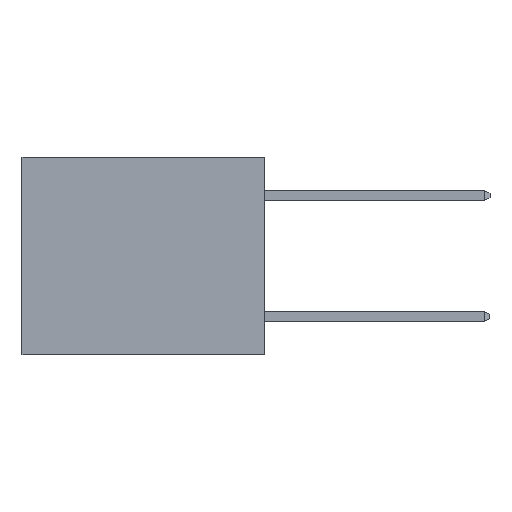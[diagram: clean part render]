
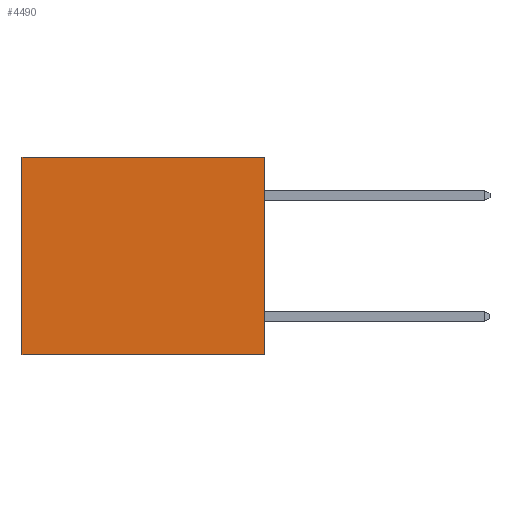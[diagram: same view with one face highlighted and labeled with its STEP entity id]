
A CAD part, left-side view. The second image highlights one B-rep face of the part: STEP entity #4490.
In plain terms, the highlighted planar face has unit normal (-1, 0, 0).
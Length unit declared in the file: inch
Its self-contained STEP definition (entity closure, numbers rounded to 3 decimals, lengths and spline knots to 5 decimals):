
#353 = CARTESIAN_POINT ( 'NONE',  ( 0.3165, 0., -0.49 ) ) ;
#411 = FACE_OUTER_BOUND ( 'NONE', #10438, .T. ) ;
#533 = EDGE_CURVE ( 'NONE', #697, #10059, #6266, .T. ) ;
#611 = AXIS2_PLACEMENT_3D ( 'NONE', #3777, #4558, #1979 ) ;
#697 = VERTEX_POINT ( 'NONE', #9895 ) ;
#712 = DIRECTION ( 'NONE',  ( 0., 1., 0. ) ) ;
#1979 = DIRECTION ( 'NONE',  ( 0., 0., -1. ) ) ;
#2061 = DIRECTION ( 'NONE',  ( 0., 0., -1. ) ) ;
#2136 = VECTOR ( 'NONE', #2906, 39.37008 ) ;
#2797 = CARTESIAN_POINT ( 'NONE',  ( 0.3165, 0.6, 0. ) ) ;
#2906 = DIRECTION ( 'NONE',  ( 0., 1., 0. ) ) ;
#2967 = PLANE ( 'NONE',  #611 ) ;
#3192 = LINE ( 'NONE', #7329, #3478 ) ;
#3478 = VECTOR ( 'NONE', #2061, 39.37008 ) ;
#3777 = CARTESIAN_POINT ( 'NONE',  ( 0.3165, 0., -0.49 ) ) ;
#3901 = VECTOR ( 'NONE', #712, 39.37008 ) ;
#4215 = ORIENTED_EDGE ( 'NONE', *, *, #11050, .T. ) ;
#4490 = ADVANCED_FACE ( 'NONE', ( #411 ), #2967, .F. ) ;
#4558 = DIRECTION ( 'NONE',  ( 1., 0., 0. ) ) ;
#4813 = VERTEX_POINT ( 'NONE', #8551 ) ;
#5181 = LINE ( 'NONE', #7562, #5321 ) ;
#5243 = ORIENTED_EDGE ( 'NONE', *, *, #533, .T. ) ;
#5321 = VECTOR ( 'NONE', #7449, 39.37008 ) ;
#5343 = CARTESIAN_POINT ( 'NONE',  ( 0.3165, 0.6, -0.49 ) ) ;
#6015 = VERTEX_POINT ( 'NONE', #5343 ) ;
#6266 = LINE ( 'NONE', #8591, #3901 ) ;
#6813 = LINE ( 'NONE', #353, #2136 ) ;
#7329 = CARTESIAN_POINT ( 'NONE',  ( 0.3165, 0., -0.49 ) ) ;
#7449 = DIRECTION ( 'NONE',  ( 0., 0., -1. ) ) ;
#7508 = EDGE_CURVE ( 'NONE', #4813, #6015, #6813, .T. ) ;
#7562 = CARTESIAN_POINT ( 'NONE',  ( 0.3165, 0.6, -0.49 ) ) ;
#7595 = ORIENTED_EDGE ( 'NONE', *, *, #7508, .F. ) ;
#8362 = EDGE_CURVE ( 'NONE', #697, #4813, #3192, .T. ) ;
#8551 = CARTESIAN_POINT ( 'NONE',  ( 0.3165, 0., -0.49 ) ) ;
#8591 = CARTESIAN_POINT ( 'NONE',  ( 0.3165, 0., 0. ) ) ;
#9895 = CARTESIAN_POINT ( 'NONE',  ( 0.3165, 0., 0. ) ) ;
#10059 = VERTEX_POINT ( 'NONE', #2797 ) ;
#10438 = EDGE_LOOP ( 'NONE', ( #4215, #7595, #10615, #5243 ) ) ;
#10615 = ORIENTED_EDGE ( 'NONE', *, *, #8362, .F. ) ;
#11050 = EDGE_CURVE ( 'NONE', #10059, #6015, #5181, .T. ) ;
